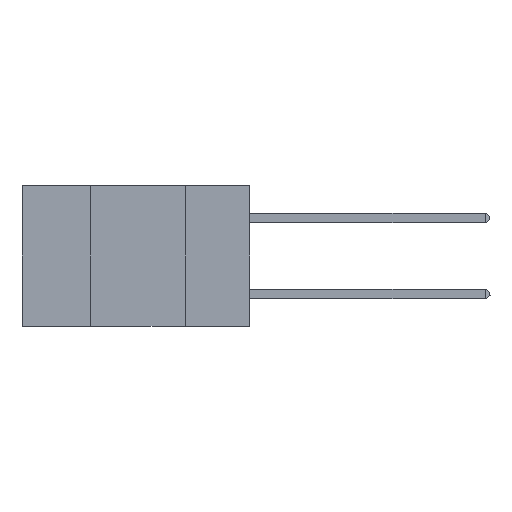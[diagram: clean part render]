
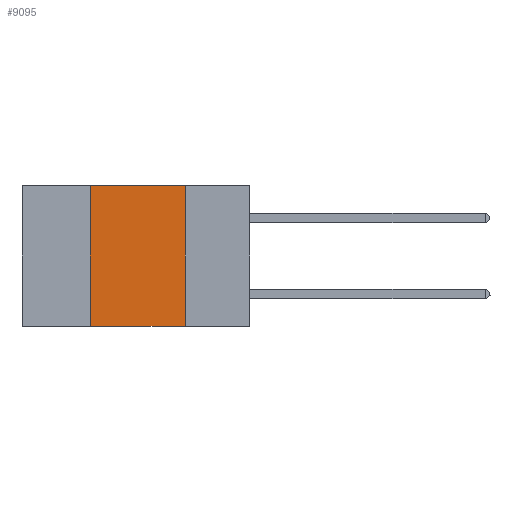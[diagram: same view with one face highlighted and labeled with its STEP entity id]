
A CAD part, left-side view. The second image highlights one B-rep face of the part: STEP entity #9095.
In plain terms, the highlighted planar face has unit normal (-1, 0, 0).
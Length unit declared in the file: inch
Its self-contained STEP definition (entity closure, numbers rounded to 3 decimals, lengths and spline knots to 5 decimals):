
#292 = VERTEX_POINT ( 'NONE', #8747 ) ;
#721 = EDGE_CURVE ( 'NONE', #11373, #2670, #16409, .T. ) ;
#1918 = CARTESIAN_POINT ( 'NONE',  ( 0., 0.42, 0. ) ) ;
#1983 = DIRECTION ( 'NONE',  ( 0., 0., 1. ) ) ;
#2665 = ORIENTED_EDGE ( 'NONE', *, *, #11989, .F. ) ;
#2670 = VERTEX_POINT ( 'NONE', #8739 ) ;
#2785 = VERTEX_POINT ( 'NONE', #14384 ) ;
#2839 = CARTESIAN_POINT ( 'NONE',  ( 0., 0.6, -0.37 ) ) ;
#3869 = ORIENTED_EDGE ( 'NONE', *, *, #5285, .F. ) ;
#4636 = ORIENTED_EDGE ( 'NONE', *, *, #721, .F. ) ;
#4645 = DIRECTION ( 'NONE',  ( 0., 0., -1. ) ) ;
#5285 = EDGE_CURVE ( 'NONE', #2670, #292, #8134, .T. ) ;
#5598 = LINE ( 'NONE', #7448, #10673 ) ;
#7448 = CARTESIAN_POINT ( 'NONE',  ( 0., 0.17, 0. ) ) ;
#7537 = FACE_OUTER_BOUND ( 'NONE', #9036, .T. ) ;
#8134 = LINE ( 'NONE', #10215, #14653 ) ;
#8593 = AXIS2_PLACEMENT_3D ( 'NONE', #16263, #14850, #4645 ) ;
#8739 = CARTESIAN_POINT ( 'NONE',  ( 0., 0.42, 0. ) ) ;
#8747 = CARTESIAN_POINT ( 'NONE',  ( 0., 0.17, 0. ) ) ;
#9036 = EDGE_LOOP ( 'NONE', ( #2665, #3869, #4636, #15505 ) ) ;
#9095 = ADVANCED_FACE ( 'NONE', ( #7537 ), #9750, .F. ) ;
#9750 = PLANE ( 'NONE',  #8593 ) ;
#10215 = CARTESIAN_POINT ( 'NONE',  ( 0., 0.6, 0. ) ) ;
#10673 = VECTOR ( 'NONE', #16672, 39.37008 ) ;
#10763 = CARTESIAN_POINT ( 'NONE',  ( 0., 0.42, -0.37 ) ) ;
#11373 = VERTEX_POINT ( 'NONE', #10763 ) ;
#11989 = EDGE_CURVE ( 'NONE', #292, #2785, #5598, .T. ) ;
#13004 = VECTOR ( 'NONE', #1983, 39.37008 ) ;
#13274 = EDGE_CURVE ( 'NONE', #11373, #2785, #15721, .T. ) ;
#14384 = CARTESIAN_POINT ( 'NONE',  ( 0., 0.17, -0.37 ) ) ;
#14470 = DIRECTION ( 'NONE',  ( 0., -1., 0. ) ) ;
#14653 = VECTOR ( 'NONE', #15442, 39.37008 ) ;
#14850 = DIRECTION ( 'NONE',  ( 1., 0., 0. ) ) ;
#15321 = VECTOR ( 'NONE', #14470, 39.37008 ) ;
#15442 = DIRECTION ( 'NONE',  ( 0., -1., 0. ) ) ;
#15505 = ORIENTED_EDGE ( 'NONE', *, *, #13274, .T. ) ;
#15721 = LINE ( 'NONE', #2839, #15321 ) ;
#16263 = CARTESIAN_POINT ( 'NONE',  ( 0., 0.6, 0. ) ) ;
#16409 = LINE ( 'NONE', #1918, #13004 ) ;
#16672 = DIRECTION ( 'NONE',  ( 0., 0., -1. ) ) ;
